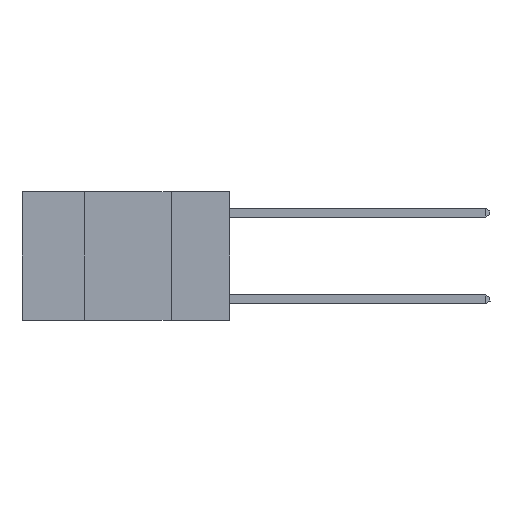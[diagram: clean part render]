
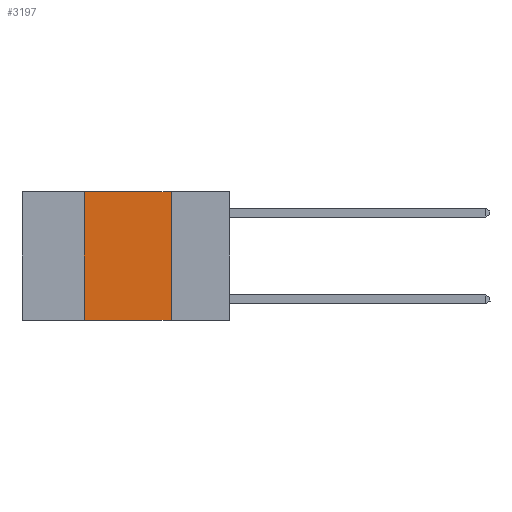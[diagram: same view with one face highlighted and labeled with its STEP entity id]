
A CAD part, left-side view. The second image highlights one B-rep face of the part: STEP entity #3197.
In plain terms, the highlighted planar face has unit normal (-1, 0, 0).
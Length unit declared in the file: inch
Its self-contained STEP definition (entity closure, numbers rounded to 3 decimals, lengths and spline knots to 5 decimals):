
#68 = PLANE ( 'NONE',  #8303 ) ;
#464 = DIRECTION ( 'NONE',  ( 0., 0., 1. ) ) ;
#556 = VERTEX_POINT ( 'NONE', #9949 ) ;
#742 = ORIENTED_EDGE ( 'NONE', *, *, #1359, .F. ) ;
#1184 = ORIENTED_EDGE ( 'NONE', *, *, #7482, .F. ) ;
#1359 = EDGE_CURVE ( 'NONE', #1682, #556, #4914, .T. ) ;
#1682 = VERTEX_POINT ( 'NONE', #6062 ) ;
#1732 = DIRECTION ( 'NONE',  ( 1., 0., 0. ) ) ;
#2242 = EDGE_CURVE ( 'NONE', #8939, #8037, #9585, .T. ) ;
#2468 = LINE ( 'NONE', #6312, #6663 ) ;
#3103 = FACE_OUTER_BOUND ( 'NONE', #7603, .T. ) ;
#3197 = ADVANCED_FACE ( 'NONE', ( #3103 ), #68, .F. ) ;
#4004 = CARTESIAN_POINT ( 'NONE',  ( 0., 0.42, -0.37 ) ) ;
#4324 = ORIENTED_EDGE ( 'NONE', *, *, #10142, .F. ) ;
#4653 = VECTOR ( 'NONE', #10434, 39.37008 ) ;
#4763 = CARTESIAN_POINT ( 'NONE',  ( 0., 0.6, -0.37 ) ) ;
#4914 = LINE ( 'NONE', #10478, #4653 ) ;
#5363 = LINE ( 'NONE', #10500, #7269 ) ;
#5926 = CARTESIAN_POINT ( 'NONE',  ( 0., 0.6, 0. ) ) ;
#6062 = CARTESIAN_POINT ( 'NONE',  ( 0., 0.42, 0. ) ) ;
#6312 = CARTESIAN_POINT ( 'NONE',  ( 0., 0.42, 0. ) ) ;
#6504 = ORIENTED_EDGE ( 'NONE', *, *, #2242, .T. ) ;
#6663 = VECTOR ( 'NONE', #464, 39.37008 ) ;
#7220 = DIRECTION ( 'NONE',  ( 0., -1., 0. ) ) ;
#7269 = VECTOR ( 'NONE', #8136, 39.37008 ) ;
#7482 = EDGE_CURVE ( 'NONE', #556, #8037, #5363, .T. ) ;
#7555 = DIRECTION ( 'NONE',  ( 0., 0., -1. ) ) ;
#7603 = EDGE_LOOP ( 'NONE', ( #1184, #742, #4324, #6504 ) ) ;
#8037 = VERTEX_POINT ( 'NONE', #8834 ) ;
#8136 = DIRECTION ( 'NONE',  ( 0., 0., -1. ) ) ;
#8303 = AXIS2_PLACEMENT_3D ( 'NONE', #5926, #1732, #7555 ) ;
#8834 = CARTESIAN_POINT ( 'NONE',  ( 0., 0.17, -0.37 ) ) ;
#8939 = VERTEX_POINT ( 'NONE', #4004 ) ;
#9341 = VECTOR ( 'NONE', #7220, 39.37008 ) ;
#9585 = LINE ( 'NONE', #4763, #9341 ) ;
#9949 = CARTESIAN_POINT ( 'NONE',  ( 0., 0.17, 0. ) ) ;
#10142 = EDGE_CURVE ( 'NONE', #8939, #1682, #2468, .T. ) ;
#10434 = DIRECTION ( 'NONE',  ( 0., -1., 0. ) ) ;
#10478 = CARTESIAN_POINT ( 'NONE',  ( 0., 0.6, 0. ) ) ;
#10500 = CARTESIAN_POINT ( 'NONE',  ( 0., 0.17, 0. ) ) ;
